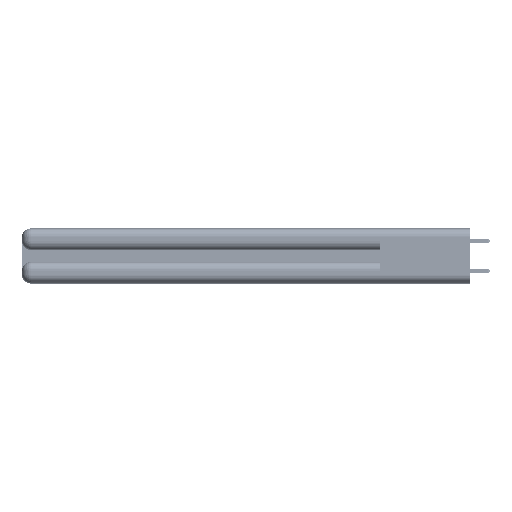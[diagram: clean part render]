
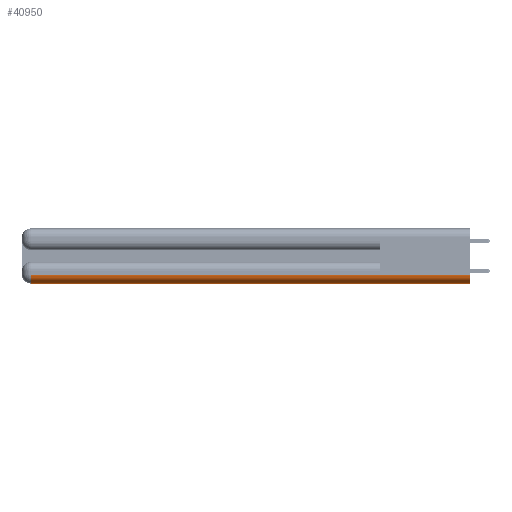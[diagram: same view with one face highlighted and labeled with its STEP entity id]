
A CAD part, left-side view. The second image highlights one B-rep face of the part: STEP entity #40950.
In plain terms, the highlighted cylindrical face has radius 1.524 mm (diameter 3.048 mm), a partial arc.
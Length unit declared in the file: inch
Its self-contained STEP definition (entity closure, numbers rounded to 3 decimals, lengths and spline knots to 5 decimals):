
#3616 = ORIENTED_EDGE ( 'NONE', *, *, #25793, .F. ) ;
#3877 = DIRECTION ( 'NONE',  ( 0., 1., 0. ) ) ;
#8191 = VERTEX_POINT ( 'NONE', #50317 ) ;
#8367 = CARTESIAN_POINT ( 'NONE',  ( 0., 0., 0.06 ) ) ;
#9629 = VECTOR ( 'NONE', #10254, 39.37008 ) ;
#9668 = ORIENTED_EDGE ( 'NONE', *, *, #52340, .F. ) ;
#10254 = DIRECTION ( 'NONE',  ( 0., -1., 0. ) ) ;
#10333 = DIRECTION ( 'NONE',  ( 0., 1., 0. ) ) ;
#14915 = CARTESIAN_POINT ( 'NONE',  ( 0.06, 0., 0.06 ) ) ;
#18996 = CARTESIAN_POINT ( 'NONE',  ( 0.06, 2.94, 0.06 ) ) ;
#21149 = CIRCLE ( 'NONE', #27586, 0.06 ) ;
#21928 = AXIS2_PLACEMENT_3D ( 'NONE', #14915, #34401, #22915 ) ;
#22623 = FACE_OUTER_BOUND ( 'NONE', #47405, .T. ) ;
#22915 = DIRECTION ( 'NONE',  ( 0., 0., 1. ) ) ;
#23861 = ORIENTED_EDGE ( 'NONE', *, *, #25052, .F. ) ;
#24834 = CARTESIAN_POINT ( 'NONE',  ( 0.06, 2.94, 0. ) ) ;
#25052 = EDGE_CURVE ( 'NONE', #39351, #8191, #21149, .T. ) ;
#25609 = DIRECTION ( 'NONE',  ( 0., 0., 1. ) ) ;
#25793 = EDGE_CURVE ( 'NONE', #39809, #39351, #44515, .T. ) ;
#26414 = CYLINDRICAL_SURFACE ( 'NONE', #21928, 0.06 ) ;
#27586 = AXIS2_PLACEMENT_3D ( 'NONE', #45846, #49932, #25609 ) ;
#27801 = ORIENTED_EDGE ( 'NONE', *, *, #29821, .F. ) ;
#29821 = EDGE_CURVE ( 'NONE', #8191, #43638, #41908, .T. ) ;
#30281 = CIRCLE ( 'NONE', #39937, 0.06 ) ;
#32671 = CARTESIAN_POINT ( 'NONE',  ( 0.06, 3., 0. ) ) ;
#34401 = DIRECTION ( 'NONE',  ( 0., 1., 0. ) ) ;
#38909 = CARTESIAN_POINT ( 'NONE',  ( 0., 0., 0.06 ) ) ;
#39351 = VERTEX_POINT ( 'NONE', #8367 ) ;
#39809 = VERTEX_POINT ( 'NONE', #51217 ) ;
#39937 = AXIS2_PLACEMENT_3D ( 'NONE', #18996, #10333, #51630 ) ;
#39960 = VECTOR ( 'NONE', #3877, 39.37008 ) ;
#40950 = ADVANCED_FACE ( 'NONE', ( #22623 ), #26414, .T. ) ;
#41908 = LINE ( 'NONE', #32671, #39960 ) ;
#43638 = VERTEX_POINT ( 'NONE', #24834 ) ;
#44515 = LINE ( 'NONE', #38909, #9629 ) ;
#45846 = CARTESIAN_POINT ( 'NONE',  ( 0.06, 0., 0.06 ) ) ;
#47405 = EDGE_LOOP ( 'NONE', ( #23861, #3616, #9668, #27801 ) ) ;
#49932 = DIRECTION ( 'NONE',  ( 0., -1., 0. ) ) ;
#50317 = CARTESIAN_POINT ( 'NONE',  ( 0.06, 0., 0. ) ) ;
#51217 = CARTESIAN_POINT ( 'NONE',  ( 0., 2.94, 0.06 ) ) ;
#51630 = DIRECTION ( 'NONE',  ( 0., 0., 1. ) ) ;
#52340 = EDGE_CURVE ( 'NONE', #43638, #39809, #30281, .T. ) ;
